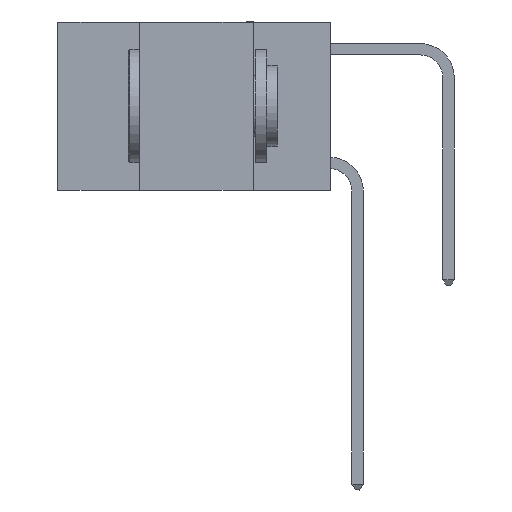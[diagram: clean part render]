
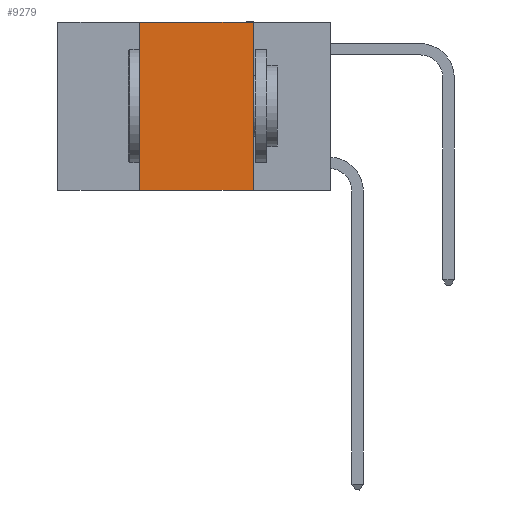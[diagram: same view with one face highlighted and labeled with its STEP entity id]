
A CAD part, left-side view. The second image highlights one B-rep face of the part: STEP entity #9279.
In plain terms, the highlighted planar face has unit normal (-1, 0, 0).
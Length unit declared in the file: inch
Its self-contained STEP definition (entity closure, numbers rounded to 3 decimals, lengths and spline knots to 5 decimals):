
#1073 = LINE ( 'NONE', #22566, #15692 ) ;
#3217 = CARTESIAN_POINT ( 'NONE',  ( 0., 0.6, 0. ) ) ;
#3240 = CARTESIAN_POINT ( 'NONE',  ( 0., 0.17, 0. ) ) ;
#3378 = LINE ( 'NONE', #3217, #18118 ) ;
#3892 = ORIENTED_EDGE ( 'NONE', *, *, #9519, .T. ) ;
#4944 = CARTESIAN_POINT ( 'NONE',  ( 0., 0.6, -0.37 ) ) ;
#9279 = ADVANCED_FACE ( 'NONE', ( #11467 ), #18332, .F. ) ;
#9519 = EDGE_CURVE ( 'NONE', #22456, #23829, #26746, .T. ) ;
#9670 = VECTOR ( 'NONE', #17560, 39.37008 ) ;
#11467 = FACE_OUTER_BOUND ( 'NONE', #25512, .T. ) ;
#13435 = DIRECTION ( 'NONE',  ( 0., 0., 1. ) ) ;
#13737 = CARTESIAN_POINT ( 'NONE',  ( 0., 0.42, -0.37 ) ) ;
#14593 = DIRECTION ( 'NONE',  ( 0., -1., 0. ) ) ;
#15692 = VECTOR ( 'NONE', #13435, 39.37008 ) ;
#16007 = ORIENTED_EDGE ( 'NONE', *, *, #19054, .F. ) ;
#17094 = ORIENTED_EDGE ( 'NONE', *, *, #26359, .F. ) ;
#17560 = DIRECTION ( 'NONE',  ( 0., 0., -1. ) ) ;
#18033 = VECTOR ( 'NONE', #14593, 39.37008 ) ;
#18118 = VECTOR ( 'NONE', #25373, 39.37008 ) ;
#18158 = CARTESIAN_POINT ( 'NONE',  ( 0., 0.6, 0. ) ) ;
#18277 = AXIS2_PLACEMENT_3D ( 'NONE', #18158, #25979, #18485 ) ;
#18332 = PLANE ( 'NONE',  #18277 ) ;
#18485 = DIRECTION ( 'NONE',  ( 0., 0., -1. ) ) ;
#19054 = EDGE_CURVE ( 'NONE', #21835, #23829, #27320, .T. ) ;
#21036 = CARTESIAN_POINT ( 'NONE',  ( 0., 0.17, -0.37 ) ) ;
#21103 = VERTEX_POINT ( 'NONE', #30971 ) ;
#21835 = VERTEX_POINT ( 'NONE', #27364 ) ;
#22456 = VERTEX_POINT ( 'NONE', #13737 ) ;
#22566 = CARTESIAN_POINT ( 'NONE',  ( 0., 0.42, 0. ) ) ;
#23829 = VERTEX_POINT ( 'NONE', #21036 ) ;
#25373 = DIRECTION ( 'NONE',  ( 0., -1., 0. ) ) ;
#25512 = EDGE_LOOP ( 'NONE', ( #16007, #17094, #30166, #3892 ) ) ;
#25979 = DIRECTION ( 'NONE',  ( 1., 0., 0. ) ) ;
#26359 = EDGE_CURVE ( 'NONE', #21103, #21835, #3378, .T. ) ;
#26746 = LINE ( 'NONE', #4944, #18033 ) ;
#27320 = LINE ( 'NONE', #3240, #9670 ) ;
#27364 = CARTESIAN_POINT ( 'NONE',  ( 0., 0.17, 0. ) ) ;
#30166 = ORIENTED_EDGE ( 'NONE', *, *, #31236, .F. ) ;
#30971 = CARTESIAN_POINT ( 'NONE',  ( 0., 0.42, 0. ) ) ;
#31236 = EDGE_CURVE ( 'NONE', #22456, #21103, #1073, .T. ) ;
